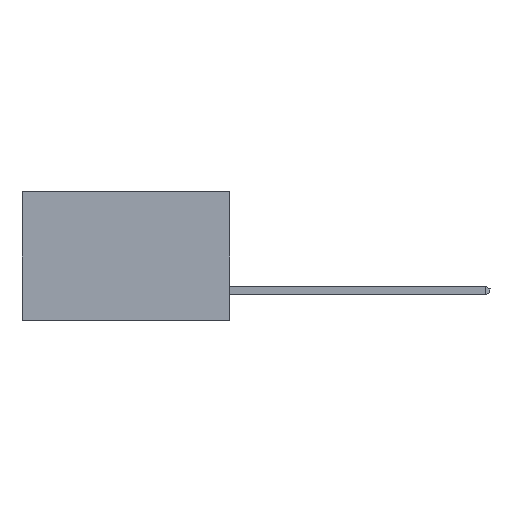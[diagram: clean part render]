
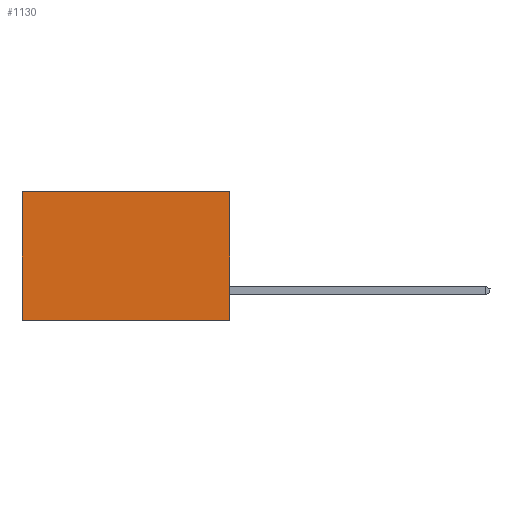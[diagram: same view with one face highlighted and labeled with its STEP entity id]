
A CAD part, left-side view. The second image highlights one B-rep face of the part: STEP entity #1130.
In plain terms, the highlighted planar face has unit normal (-1, 0, 0).
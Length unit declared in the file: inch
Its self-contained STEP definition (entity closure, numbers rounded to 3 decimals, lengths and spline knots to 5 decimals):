
#435 = ORIENTED_EDGE ( 'NONE', *, *, #2805, .F. ) ;
#1037 = CARTESIAN_POINT ( 'NONE',  ( 0.2615, 0., -0.37 ) ) ;
#1074 = DIRECTION ( 'NONE',  ( 0., 1., 0. ) ) ;
#1130 = ADVANCED_FACE ( 'NONE', ( #4857 ), #8145, .F. ) ;
#1689 = VERTEX_POINT ( 'NONE', #3171 ) ;
#1738 = VERTEX_POINT ( 'NONE', #4326 ) ;
#1800 = CARTESIAN_POINT ( 'NONE',  ( 0.2615, 0., 0. ) ) ;
#1899 = LINE ( 'NONE', #8158, #3561 ) ;
#2220 = CARTESIAN_POINT ( 'NONE',  ( 0.2615, 0., -0.37 ) ) ;
#2805 = EDGE_CURVE ( 'NONE', #6981, #1738, #8216, .T. ) ;
#2961 = DIRECTION ( 'NONE',  ( 0., 0., -1. ) ) ;
#3038 = LINE ( 'NONE', #7761, #5995 ) ;
#3171 = CARTESIAN_POINT ( 'NONE',  ( 0.2615, 0.6, -0.37 ) ) ;
#3405 = EDGE_CURVE ( 'NONE', #6981, #4528, #5680, .T. ) ;
#3561 = VECTOR ( 'NONE', #4996, 39.37008 ) ;
#3635 = CARTESIAN_POINT ( 'NONE',  ( 0.2615, 0.6, 0. ) ) ;
#3828 = ORIENTED_EDGE ( 'NONE', *, *, #3405, .T. ) ;
#3889 = ORIENTED_EDGE ( 'NONE', *, *, #8061, .T. ) ;
#4326 = CARTESIAN_POINT ( 'NONE',  ( 0.2615, 0., -0.37 ) ) ;
#4524 = CARTESIAN_POINT ( 'NONE',  ( 0.2615, 0., 0. ) ) ;
#4528 = VERTEX_POINT ( 'NONE', #3635 ) ;
#4695 = EDGE_CURVE ( 'NONE', #1738, #1689, #3038, .T. ) ;
#4857 = FACE_OUTER_BOUND ( 'NONE', #7638, .T. ) ;
#4996 = DIRECTION ( 'NONE',  ( 0., 0., -1. ) ) ;
#5680 = LINE ( 'NONE', #1800, #7241 ) ;
#5995 = VECTOR ( 'NONE', #8294, 39.37008 ) ;
#6981 = VERTEX_POINT ( 'NONE', #4524 ) ;
#7241 = VECTOR ( 'NONE', #1074, 39.37008 ) ;
#7440 = DIRECTION ( 'NONE',  ( 0., 0., -1. ) ) ;
#7486 = DIRECTION ( 'NONE',  ( 1., 0., 0. ) ) ;
#7638 = EDGE_LOOP ( 'NONE', ( #3889, #8326, #435, #3828 ) ) ;
#7761 = CARTESIAN_POINT ( 'NONE',  ( 0.2615, 0., -0.37 ) ) ;
#7781 = AXIS2_PLACEMENT_3D ( 'NONE', #2220, #7486, #2961 ) ;
#8061 = EDGE_CURVE ( 'NONE', #4528, #1689, #1899, .T. ) ;
#8145 = PLANE ( 'NONE',  #7781 ) ;
#8158 = CARTESIAN_POINT ( 'NONE',  ( 0.2615, 0.6, -0.37 ) ) ;
#8216 = LINE ( 'NONE', #1037, #8228 ) ;
#8228 = VECTOR ( 'NONE', #7440, 39.37008 ) ;
#8294 = DIRECTION ( 'NONE',  ( 0., 1., 0. ) ) ;
#8326 = ORIENTED_EDGE ( 'NONE', *, *, #4695, .F. ) ;
